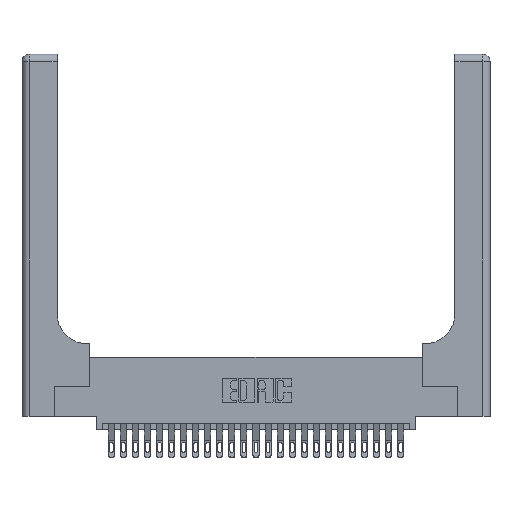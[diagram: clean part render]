
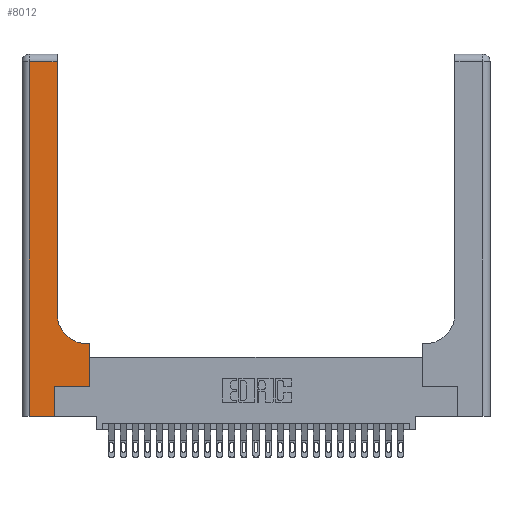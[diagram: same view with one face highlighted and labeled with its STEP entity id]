
A CAD part, top view. The second image highlights one B-rep face of the part: STEP entity #8012.
In plain terms, the highlighted planar face has unit normal (0, 0, 1).
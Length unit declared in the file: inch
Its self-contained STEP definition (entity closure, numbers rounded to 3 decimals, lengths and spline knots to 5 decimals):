
#404 = EDGE_CURVE ( 'NONE', #5196, #16158, #3864, .T. ) ;
#601 = ORIENTED_EDGE ( 'NONE', *, *, #8063, .T. ) ;
#1161 = EDGE_CURVE ( 'NONE', #20993, #5196, #20781, .T. ) ;
#1187 = CARTESIAN_POINT ( 'NONE',  ( 0.06, 2.94, 0.37 ) ) ;
#1257 = ORIENTED_EDGE ( 'NONE', *, *, #18481, .T. ) ;
#1278 = CARTESIAN_POINT ( 'NONE',  ( 0., 0., 0.37 ) ) ;
#1464 = PLANE ( 'NONE',  #4027 ) ;
#1984 = CARTESIAN_POINT ( 'NONE',  ( 0.06, 3., 0.37 ) ) ;
#2083 = ORIENTED_EDGE ( 'NONE', *, *, #20642, .T. ) ;
#2280 = LINE ( 'NONE', #1278, #7350 ) ;
#2395 = DIRECTION ( 'NONE',  ( 0., 1., 0. ) ) ;
#2795 = VERTEX_POINT ( 'NONE', #27330 ) ;
#3864 = LINE ( 'NONE', #10816, #9841 ) ;
#4027 = AXIS2_PLACEMENT_3D ( 'NONE', #27037, #26948, #18595 ) ;
#4409 = ORIENTED_EDGE ( 'NONE', *, *, #404, .T. ) ;
#4869 = CARTESIAN_POINT ( 'NONE',  ( 0.269, 0., 0.37 ) ) ;
#5196 = VERTEX_POINT ( 'NONE', #12656 ) ;
#5363 = DIRECTION ( 'NONE',  ( -1., 0., 0. ) ) ;
#5825 = VECTOR ( 'NONE', #5363, 39.37008 ) ;
#5957 = CARTESIAN_POINT ( 'NONE',  ( 0.5585, 0.25, 0.37 ) ) ;
#6458 = DIRECTION ( 'NONE',  ( 1., 0., 0. ) ) ;
#6509 = VECTOR ( 'NONE', #25564, 39.37008 ) ;
#7350 = VECTOR ( 'NONE', #10052, 39.37008 ) ;
#7707 = LINE ( 'NONE', #1984, #10661 ) ;
#8009 = FACE_OUTER_BOUND ( 'NONE', #19409, .T. ) ;
#8012 = ADVANCED_FACE ( 'NONE', ( #8009 ), #1464, .F. ) ;
#8063 = EDGE_CURVE ( 'NONE', #2795, #20993, #2280, .T. ) ;
#9027 = VERTEX_POINT ( 'NONE', #10637 ) ;
#9471 = VECTOR ( 'NONE', #2395, 39.37008 ) ;
#9841 = VECTOR ( 'NONE', #6458, 39.37008 ) ;
#10052 = DIRECTION ( 'NONE',  ( 1., 0., 0. ) ) ;
#10188 = CARTESIAN_POINT ( 'NONE',  ( 0.2915, 0.85, 0.37 ) ) ;
#10637 = CARTESIAN_POINT ( 'NONE',  ( 0.2915, 2.94, 0.37 ) ) ;
#10661 = VECTOR ( 'NONE', #27298, 39.37008 ) ;
#10816 = CARTESIAN_POINT ( 'NONE',  ( 0.269, 0.25, 0.37 ) ) ;
#10868 = CIRCLE ( 'NONE', #15736, 0.25 ) ;
#11235 = ORIENTED_EDGE ( 'NONE', *, *, #26208, .T. ) ;
#11623 = VERTEX_POINT ( 'NONE', #21750 ) ;
#11719 = CARTESIAN_POINT ( 'NONE',  ( 0.5415, 0.85, 0.37 ) ) ;
#12561 = EDGE_CURVE ( 'NONE', #19273, #2795, #7707, .T. ) ;
#12656 = CARTESIAN_POINT ( 'NONE',  ( 0.269, 0.25, 0.37 ) ) ;
#12850 = LINE ( 'NONE', #19857, #27147 ) ;
#13848 = DIRECTION ( 'NONE',  ( 0., 0., -1. ) ) ;
#14874 = ORIENTED_EDGE ( 'NONE', *, *, #12561, .T. ) ;
#15626 = ORIENTED_EDGE ( 'NONE', *, *, #1161, .T. ) ;
#15736 = AXIS2_PLACEMENT_3D ( 'NONE', #11719, #13848, #15987 ) ;
#15987 = DIRECTION ( 'NONE',  ( 1., 0., 0. ) ) ;
#16158 = VERTEX_POINT ( 'NONE', #5957 ) ;
#16786 = LINE ( 'NONE', #25654, #6509 ) ;
#17095 = LINE ( 'NONE', #18049, #5825 ) ;
#18049 = CARTESIAN_POINT ( 'NONE',  ( 0.2915, 0.6, 0.37 ) ) ;
#18061 = CARTESIAN_POINT ( 'NONE',  ( 0.2915, 3., 0.37 ) ) ;
#18481 = EDGE_CURVE ( 'NONE', #9027, #19273, #12850, .T. ) ;
#18595 = DIRECTION ( 'NONE',  ( -1., 0., 0. ) ) ;
#19273 = VERTEX_POINT ( 'NONE', #1187 ) ;
#19409 = EDGE_LOOP ( 'NONE', ( #11235, #1257, #14874, #601, #15626, #4409, #21916, #2083, #23554 ) ) ;
#19857 = CARTESIAN_POINT ( 'NONE',  ( 0., 2.94, 0.37 ) ) ;
#20180 = VERTEX_POINT ( 'NONE', #10188 ) ;
#20318 = EDGE_CURVE ( 'NONE', #16158, #11623, #16786, .T. ) ;
#20324 = DIRECTION ( 'NONE',  ( 0., 1., 0. ) ) ;
#20642 = EDGE_CURVE ( 'NONE', #11623, #24119, #17095, .T. ) ;
#20781 = LINE ( 'NONE', #4869, #9471 ) ;
#20993 = VERTEX_POINT ( 'NONE', #23320 ) ;
#21750 = CARTESIAN_POINT ( 'NONE',  ( 0.5585, 0.6, 0.37 ) ) ;
#21895 = DIRECTION ( 'NONE',  ( -1., 0., 0. ) ) ;
#21916 = ORIENTED_EDGE ( 'NONE', *, *, #20318, .T. ) ;
#23320 = CARTESIAN_POINT ( 'NONE',  ( 0.269, 0., 0.37 ) ) ;
#23554 = ORIENTED_EDGE ( 'NONE', *, *, #26934, .T. ) ;
#24119 = VERTEX_POINT ( 'NONE', #24916 ) ;
#24916 = CARTESIAN_POINT ( 'NONE',  ( 0.5415, 0.6, 0.37 ) ) ;
#25564 = DIRECTION ( 'NONE',  ( 0., 1., 0. ) ) ;
#25654 = CARTESIAN_POINT ( 'NONE',  ( 0.5585, 0.25, 0.37 ) ) ;
#26208 = EDGE_CURVE ( 'NONE', #20180, #9027, #26860, .T. ) ;
#26860 = LINE ( 'NONE', #18061, #27178 ) ;
#26934 = EDGE_CURVE ( 'NONE', #24119, #20180, #10868, .T. ) ;
#26948 = DIRECTION ( 'NONE',  ( 0., 0., -1. ) ) ;
#27037 = CARTESIAN_POINT ( 'NONE',  ( 0., 3., 0.37 ) ) ;
#27147 = VECTOR ( 'NONE', #21895, 39.37008 ) ;
#27178 = VECTOR ( 'NONE', #20324, 39.37008 ) ;
#27298 = DIRECTION ( 'NONE',  ( 0., -1., 0. ) ) ;
#27330 = CARTESIAN_POINT ( 'NONE',  ( 0.06, 0., 0.37 ) ) ;
